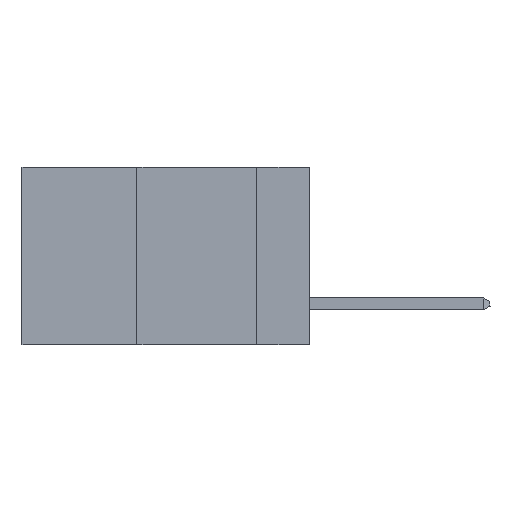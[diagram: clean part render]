
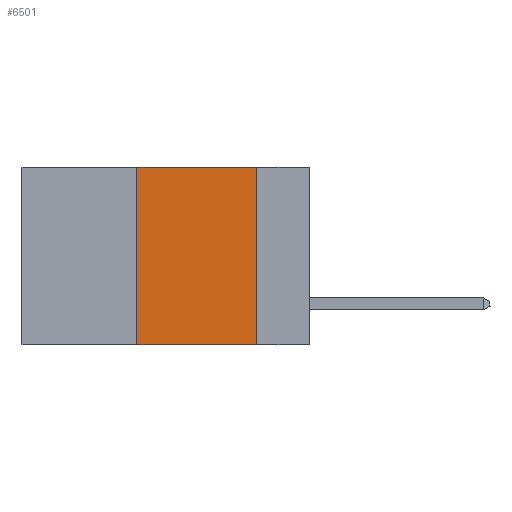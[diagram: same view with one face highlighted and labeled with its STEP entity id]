
A CAD part, left-side view. The second image highlights one B-rep face of the part: STEP entity #6501.
In plain terms, the highlighted planar face has unit normal (-1, 0, 0).
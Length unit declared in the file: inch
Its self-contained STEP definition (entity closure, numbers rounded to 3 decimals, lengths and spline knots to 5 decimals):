
#821 = LINE ( 'NONE', #14059, #9335 ) ;
#3752 = FACE_OUTER_BOUND ( 'NONE', #17432, .T. ) ;
#3792 = CARTESIAN_POINT ( 'NONE',  ( 0., 0.36, 0. ) ) ;
#6292 = ORIENTED_EDGE ( 'NONE', *, *, #24344, .F. ) ;
#6501 = ADVANCED_FACE ( 'NONE', ( #3752 ), #25249, .F. ) ;
#7804 = CARTESIAN_POINT ( 'NONE',  ( 0., 0.11, -0.37 ) ) ;
#8091 = CARTESIAN_POINT ( 'NONE',  ( 0., 0.36, -0.37 ) ) ;
#8442 = ORIENTED_EDGE ( 'NONE', *, *, #31605, .F. ) ;
#8771 = CARTESIAN_POINT ( 'NONE',  ( 0., 0.6, 0. ) ) ;
#9335 = VECTOR ( 'NONE', #16266, 39.37008 ) ;
#13058 = DIRECTION ( 'NONE',  ( 0., 0., -1. ) ) ;
#13161 = CARTESIAN_POINT ( 'NONE',  ( 0., 0.6, 0. ) ) ;
#13981 = VERTEX_POINT ( 'NONE', #7804 ) ;
#14059 = CARTESIAN_POINT ( 'NONE',  ( 0., 0.6, -0.37 ) ) ;
#15980 = VECTOR ( 'NONE', #18860, 39.37008 ) ;
#16266 = DIRECTION ( 'NONE',  ( 0., -1., 0. ) ) ;
#17432 = EDGE_LOOP ( 'NONE', ( #6292, #8442, #31077, #30486 ) ) ;
#17445 = VERTEX_POINT ( 'NONE', #25888 ) ;
#18040 = EDGE_CURVE ( 'NONE', #30997, #29250, #29018, .T. ) ;
#18127 = VECTOR ( 'NONE', #24920, 39.37008 ) ;
#18860 = DIRECTION ( 'NONE',  ( 0., 0., 1. ) ) ;
#20777 = DIRECTION ( 'NONE',  ( 0., -1., 0. ) ) ;
#22467 = CARTESIAN_POINT ( 'NONE',  ( 0., 0.11, 0. ) ) ;
#24185 = CARTESIAN_POINT ( 'NONE',  ( 0., 0.36, 0. ) ) ;
#24344 = EDGE_CURVE ( 'NONE', #17445, #13981, #29630, .T. ) ;
#24920 = DIRECTION ( 'NONE',  ( 0., 0., -1. ) ) ;
#25249 = PLANE ( 'NONE',  #27413 ) ;
#25888 = CARTESIAN_POINT ( 'NONE',  ( 0., 0.11, 0. ) ) ;
#26769 = LINE ( 'NONE', #8771, #27890 ) ;
#27413 = AXIS2_PLACEMENT_3D ( 'NONE', #13161, #30071, #13058 ) ;
#27890 = VECTOR ( 'NONE', #20777, 39.37008 ) ;
#29018 = LINE ( 'NONE', #3792, #15980 ) ;
#29250 = VERTEX_POINT ( 'NONE', #24185 ) ;
#29579 = EDGE_CURVE ( 'NONE', #30997, #13981, #821, .T. ) ;
#29630 = LINE ( 'NONE', #22467, #18127 ) ;
#30071 = DIRECTION ( 'NONE',  ( 1., 0., 0. ) ) ;
#30486 = ORIENTED_EDGE ( 'NONE', *, *, #29579, .T. ) ;
#30997 = VERTEX_POINT ( 'NONE', #8091 ) ;
#31077 = ORIENTED_EDGE ( 'NONE', *, *, #18040, .F. ) ;
#31605 = EDGE_CURVE ( 'NONE', #29250, #17445, #26769, .T. ) ;
